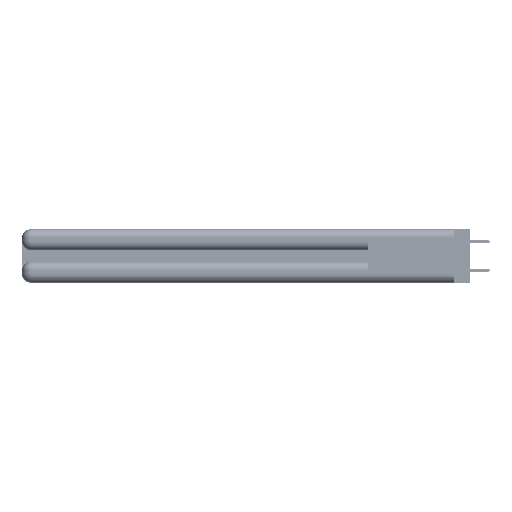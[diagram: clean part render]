
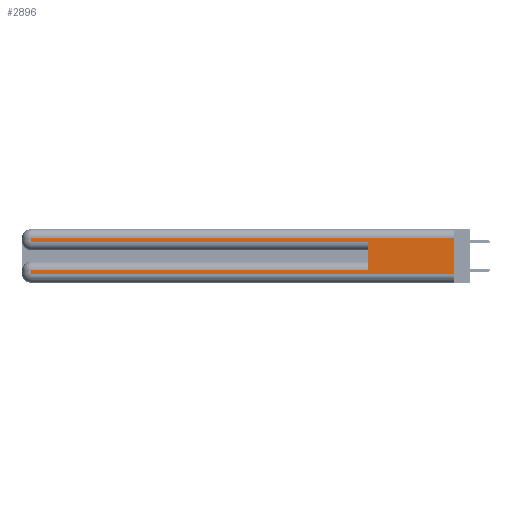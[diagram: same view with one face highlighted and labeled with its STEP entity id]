
A CAD part, left-side view. The second image highlights one B-rep face of the part: STEP entity #2896.
In plain terms, the highlighted planar face has unit normal (-1, 0, 0).
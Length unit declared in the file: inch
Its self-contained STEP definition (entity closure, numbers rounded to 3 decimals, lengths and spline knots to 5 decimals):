
#2896 = ADVANCED_FACE ( 'NONE', ( #29547 ), #12470, .F. ) ;
#3367 = CARTESIAN_POINT ( 'NONE',  ( 0., 0., 0.31 ) ) ;
#3743 = CARTESIAN_POINT ( 'NONE',  ( 0., 0., 0.31 ) ) ;
#3960 = CARTESIAN_POINT ( 'NONE',  ( 0., 0., 0.06 ) ) ;
#4173 = EDGE_CURVE ( 'NONE', #27362, #32474, #5583, .T. ) ;
#5372 = CARTESIAN_POINT ( 'NONE',  ( 0., 2.94, 0.285 ) ) ;
#5583 = LINE ( 'NONE', #3960, #26224 ) ;
#6768 = DIRECTION ( 'NONE',  ( 0., 1., 0. ) ) ;
#7813 = VERTEX_POINT ( 'NONE', #46688 ) ;
#8190 = CARTESIAN_POINT ( 'NONE',  ( 0., 0.6, 0.145 ) ) ;
#8402 = CARTESIAN_POINT ( 'NONE',  ( 0., 0., 0.06 ) ) ;
#9230 = CARTESIAN_POINT ( 'NONE',  ( 0., 0.6, 0.085 ) ) ;
#11685 = LINE ( 'NONE', #39881, #41890 ) ;
#11721 = AXIS2_PLACEMENT_3D ( 'NONE', #45451, #20901, #49540 ) ;
#12172 = DIRECTION ( 'NONE',  ( 0., -1., 0. ) ) ;
#12355 = CARTESIAN_POINT ( 'NONE',  ( 0., 2.94, 0.31 ) ) ;
#12470 = PLANE ( 'NONE',  #11721 ) ;
#12741 = VERTEX_POINT ( 'NONE', #3367 ) ;
#12975 = ORIENTED_EDGE ( 'NONE', *, *, #31774, .F. ) ;
#15275 = DIRECTION ( 'NONE',  ( 0., 0., -1. ) ) ;
#15437 = ORIENTED_EDGE ( 'NONE', *, *, #4173, .T. ) ;
#15750 = DIRECTION ( 'NONE',  ( 0., 0., -1. ) ) ;
#15757 = LINE ( 'NONE', #8190, #49692 ) ;
#16429 = LINE ( 'NONE', #35565, #47828 ) ;
#16553 = DIRECTION ( 'NONE',  ( 0., 0., 1. ) ) ;
#16812 = VERTEX_POINT ( 'NONE', #9230 ) ;
#17851 = ORIENTED_EDGE ( 'NONE', *, *, #40272, .T. ) ;
#18311 = EDGE_CURVE ( 'NONE', #7813, #27362, #11685, .T. ) ;
#18435 = VECTOR ( 'NONE', #52980, 39.37008 ) ;
#19317 = ORIENTED_EDGE ( 'NONE', *, *, #37735, .F. ) ;
#19368 = LINE ( 'NONE', #44820, #52035 ) ;
#20277 = DIRECTION ( 'NONE',  ( 0., 0., -1. ) ) ;
#20901 = DIRECTION ( 'NONE',  ( 1., 0., 0. ) ) ;
#21498 = ORIENTED_EDGE ( 'NONE', *, *, #24232, .T. ) ;
#24232 = EDGE_CURVE ( 'NONE', #44944, #40533, #26756, .T. ) ;
#25077 = CARTESIAN_POINT ( 'NONE',  ( 0., 0.6, 0.285 ) ) ;
#25787 = ORIENTED_EDGE ( 'NONE', *, *, #31527, .T. ) ;
#25910 = DIRECTION ( 'NONE',  ( 0., -1., 0. ) ) ;
#26224 = VECTOR ( 'NONE', #12172, 39.37008 ) ;
#26756 = LINE ( 'NONE', #32016, #36407 ) ;
#27362 = VERTEX_POINT ( 'NONE', #36764 ) ;
#29482 = EDGE_LOOP ( 'NONE', ( #19317, #17851, #21498, #30821, #12975, #25787, #52339, #15437 ) ) ;
#29547 = FACE_OUTER_BOUND ( 'NONE', #29482, .T. ) ;
#29837 = CARTESIAN_POINT ( 'NONE',  ( 0., 0., 0.285 ) ) ;
#30581 = VERTEX_POINT ( 'NONE', #25077 ) ;
#30821 = ORIENTED_EDGE ( 'NONE', *, *, #40517, .T. ) ;
#31527 = EDGE_CURVE ( 'NONE', #16812, #7813, #16429, .T. ) ;
#31774 = EDGE_CURVE ( 'NONE', #16812, #30581, #15757, .T. ) ;
#32016 = CARTESIAN_POINT ( 'NONE',  ( 0., 2.94, 0.37 ) ) ;
#32474 = VERTEX_POINT ( 'NONE', #8402 ) ;
#34101 = VECTOR ( 'NONE', #25910, 39.37008 ) ;
#35565 = CARTESIAN_POINT ( 'NONE',  ( 0., 0., 0.085 ) ) ;
#36407 = VECTOR ( 'NONE', #15750, 39.37008 ) ;
#36764 = CARTESIAN_POINT ( 'NONE',  ( 0., 2.94, 0.06 ) ) ;
#37735 = EDGE_CURVE ( 'NONE', #12741, #32474, #19368, .T. ) ;
#39881 = CARTESIAN_POINT ( 'NONE',  ( 0., 2.94, 0.37 ) ) ;
#40272 = EDGE_CURVE ( 'NONE', #12741, #44944, #51098, .T. ) ;
#40517 = EDGE_CURVE ( 'NONE', #40533, #30581, #45018, .T. ) ;
#40533 = VERTEX_POINT ( 'NONE', #5372 ) ;
#41890 = VECTOR ( 'NONE', #15275, 39.37008 ) ;
#44820 = CARTESIAN_POINT ( 'NONE',  ( 0., 0., 0.37 ) ) ;
#44944 = VERTEX_POINT ( 'NONE', #12355 ) ;
#45018 = LINE ( 'NONE', #29837, #34101 ) ;
#45451 = CARTESIAN_POINT ( 'NONE',  ( 0., 0., 0.37 ) ) ;
#46688 = CARTESIAN_POINT ( 'NONE',  ( 0., 2.94, 0.085 ) ) ;
#47828 = VECTOR ( 'NONE', #6768, 39.37008 ) ;
#49540 = DIRECTION ( 'NONE',  ( 0., 0., -1. ) ) ;
#49692 = VECTOR ( 'NONE', #16553, 39.37008 ) ;
#51098 = LINE ( 'NONE', #3743, #18435 ) ;
#52035 = VECTOR ( 'NONE', #20277, 39.37008 ) ;
#52339 = ORIENTED_EDGE ( 'NONE', *, *, #18311, .T. ) ;
#52980 = DIRECTION ( 'NONE',  ( 0., 1., 0. ) ) ;
